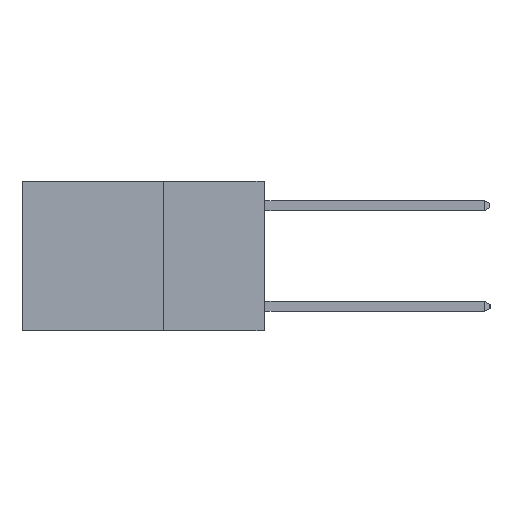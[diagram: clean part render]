
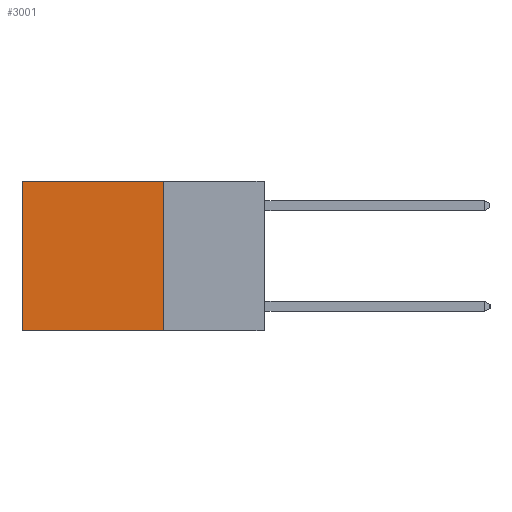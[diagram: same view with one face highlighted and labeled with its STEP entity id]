
A CAD part, left-side view. The second image highlights one B-rep face of the part: STEP entity #3001.
In plain terms, the highlighted planar face has unit normal (-1, 0, 0).
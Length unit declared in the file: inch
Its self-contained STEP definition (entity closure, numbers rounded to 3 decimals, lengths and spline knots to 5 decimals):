
#884 = DIRECTION ( 'NONE',  ( 0., 0., -1. ) ) ;
#931 = CARTESIAN_POINT ( 'NONE',  ( 0.2625, 0.6, -0.37 ) ) ;
#1034 = DIRECTION ( 'NONE',  ( 0., 1., 0. ) ) ;
#1138 = CARTESIAN_POINT ( 'NONE',  ( 0.2625, 0.25, 0. ) ) ;
#1728 = EDGE_LOOP ( 'NONE', ( #4544, #4562, #4575, #4592 ) ) ;
#2041 = CARTESIAN_POINT ( 'NONE',  ( 0.2625, 0.6, 0. ) ) ;
#2968 = CARTESIAN_POINT ( 'NONE',  ( 0.2625, 0.25, 0. ) ) ;
#3001 = ADVANCED_FACE ( 'NONE', ( #7079 ), #4801, .F. ) ;
#3032 = CARTESIAN_POINT ( 'NONE',  ( 0.2625, 0.25, -0.37 ) ) ;
#3105 = CARTESIAN_POINT ( 'NONE',  ( 0.2625, 0.25, 0. ) ) ;
#3684 = VERTEX_POINT ( 'NONE', #2041 ) ;
#4074 = DIRECTION ( 'NONE',  ( 0., 0., -1. ) ) ;
#4534 = VERTEX_POINT ( 'NONE', #3032 ) ;
#4544 = ORIENTED_EDGE ( 'NONE', *, *, #6660, .T. ) ;
#4562 = ORIENTED_EDGE ( 'NONE', *, *, #4624, .F. ) ;
#4575 = ORIENTED_EDGE ( 'NONE', *, *, #7519, .F. ) ;
#4592 = ORIENTED_EDGE ( 'NONE', *, *, #5403, .T. ) ;
#4624 = EDGE_CURVE ( 'NONE', #4534, #11023, #10071, .T. ) ;
#4801 = PLANE ( 'NONE',  #4899 ) ;
#4899 = AXIS2_PLACEMENT_3D ( 'NONE', #10401, #6542, #884 ) ;
#5403 = EDGE_CURVE ( 'NONE', #6220, #3684, #6762, .T. ) ;
#5475 = DIRECTION ( 'NONE',  ( 0., 0., -1. ) ) ;
#5599 = VECTOR ( 'NONE', #1034, 39.37008 ) ;
#6220 = VERTEX_POINT ( 'NONE', #1138 ) ;
#6506 = VECTOR ( 'NONE', #9088, 39.37008 ) ;
#6542 = DIRECTION ( 'NONE',  ( 1., 0., 0. ) ) ;
#6660 = EDGE_CURVE ( 'NONE', #3684, #11023, #7420, .T. ) ;
#6680 = CARTESIAN_POINT ( 'NONE',  ( 0.2625, 0.25, -0.37 ) ) ;
#6762 = LINE ( 'NONE', #3105, #6506 ) ;
#7079 = FACE_OUTER_BOUND ( 'NONE', #1728, .T. ) ;
#7243 = VECTOR ( 'NONE', #4074, 39.37008 ) ;
#7420 = LINE ( 'NONE', #10909, #9222 ) ;
#7519 = EDGE_CURVE ( 'NONE', #6220, #4534, #9317, .T. ) ;
#9088 = DIRECTION ( 'NONE',  ( 0., 1., 0. ) ) ;
#9222 = VECTOR ( 'NONE', #5475, 39.37008 ) ;
#9317 = LINE ( 'NONE', #2968, #7243 ) ;
#10071 = LINE ( 'NONE', #6680, #5599 ) ;
#10401 = CARTESIAN_POINT ( 'NONE',  ( 0.2625, 0.25, 0. ) ) ;
#10909 = CARTESIAN_POINT ( 'NONE',  ( 0.2625, 0.6, 0. ) ) ;
#11023 = VERTEX_POINT ( 'NONE', #931 ) ;
